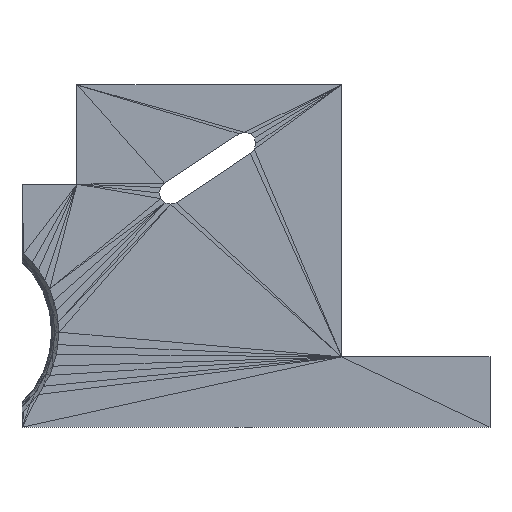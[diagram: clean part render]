
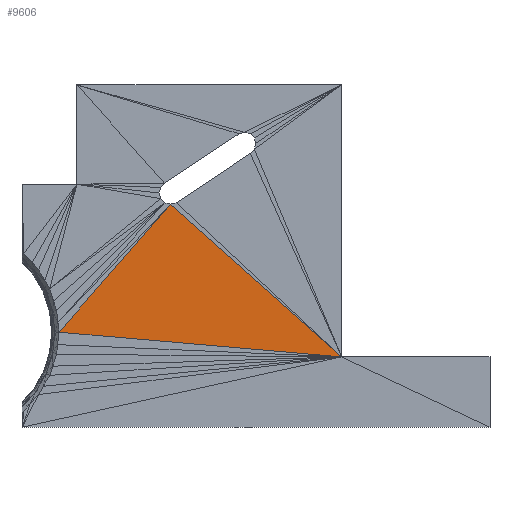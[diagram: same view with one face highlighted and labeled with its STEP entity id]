
A CAD part, top view. The second image highlights one B-rep face of the part: STEP entity #9606.
In plain terms, the highlighted planar face has unit normal (0, 0, 1).
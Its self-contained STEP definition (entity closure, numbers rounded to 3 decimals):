
#2076 = VERTEX_POINT('',#2077);
#2077 = CARTESIAN_POINT('',(12.446,-12.7,
    3.047));
#2202 = PLANE('',#2203);
#2203 = AXIS2_PLACEMENT_3D('',#2204,#2205,#2206);
#2204 = CARTESIAN_POINT('',(1.503,-2.733,
    3.047));
#2205 = DIRECTION('',(0.,0.,1.));
#2206 = DIRECTION('',(0.,1.,0.));
#2242 = EDGE_CURVE('',#2243,#2076,#2245,.T.);
#2243 = VERTEX_POINT('',#2244);
#2244 = CARTESIAN_POINT('',(-9.525,6.89,3.047
    ));
#2245 = SURFACE_CURVE('',#2246,(#2250,#2257),.PCURVE_S1.);
#2246 = LINE('',#2247,#2248);
#2247 = CARTESIAN_POINT('',(-9.525,6.89,3.047
    ));
#2248 = VECTOR('',#2249,1.);
#2249 = DIRECTION('',(0.746,-0.666,0.));
#2250 = PCURVE('',#2202,#2251);
#2251 = DEFINITIONAL_REPRESENTATION('',(#2252),#2256);
#2252 = LINE('',#2253,#2254);
#2253 = CARTESIAN_POINT('',(9.622,11.028));
#2254 = VECTOR('',#2255,1.);
#2255 = DIRECTION('',(-0.666,-0.746));
#2256 = ( GEOMETRIC_REPRESENTATION_CONTEXT(2) 
PARAMETRIC_REPRESENTATION_CONTEXT() REPRESENTATION_CONTEXT('2D SPACE',''
  ) );
#2257 = PCURVE('',#2258,#2263);
#2258 = PLANE('',#2259);
#2259 = AXIS2_PLACEMENT_3D('',#2260,#2261,#2262);
#2260 = CARTESIAN_POINT('',(-6.022,-5.922,
    3.047));
#2261 = DIRECTION('',(0.,0.,1.));
#2262 = DIRECTION('',(1.,0.,-0.));
#2263 = DEFINITIONAL_REPRESENTATION('',(#2264),#2267);
#2264 = B_SPLINE_CURVE_WITH_KNOTS('',1,(#2265,#2266),.UNSPECIFIED.,.F.,
  .F.,(2,2),(0.,29.436),.PIECEWISE_BEZIER_KNOTS.);
#2265 = CARTESIAN_POINT('',(-3.503,12.811));
#2266 = CARTESIAN_POINT('',(18.468,-6.778));
#2267 = ( GEOMETRIC_REPRESENTATION_CONTEXT(2) 
PARAMETRIC_REPRESENTATION_CONTEXT() REPRESENTATION_CONTEXT('2D SPACE',''
  ) );
#3751 = VERTEX_POINT('',#3752);
#3752 = CARTESIAN_POINT('',(-23.837,-9.525,3.047
    ));
#3766 = PLANE('',#3767);
#3767 = AXIS2_PLACEMENT_3D('',#3768,#3769,#3770);
#3768 = CARTESIAN_POINT('',(-6.131,-11.488,
    3.047));
#3769 = DIRECTION('',(0.,0.,1.));
#3770 = DIRECTION('',(0.,1.,0.));
#8823 = PLANE('',#8824);
#8824 = AXIS2_PLACEMENT_3D('',#8825,#8826,#8827);
#8825 = CARTESIAN_POINT('',(-16.915,-1.238,
    3.047));
#8826 = DIRECTION('',(0.,0.,1.));
#8827 = DIRECTION('',(1.,0.,-0.));
#9245 = EDGE_CURVE('',#3751,#2243,#9246,.T.);
#9246 = SURFACE_CURVE('',#9247,(#9251,#9258),.PCURVE_S1.);
#9247 = LINE('',#9248,#9249);
#9248 = CARTESIAN_POINT('',(-23.837,-9.525,3.047
    ));
#9249 = VECTOR('',#9250,1.);
#9250 = DIRECTION('',(0.657,0.754,0.));
#9251 = PCURVE('',#8823,#9252);
#9252 = DEFINITIONAL_REPRESENTATION('',(#9253),#9257);
#9253 = LINE('',#9254,#9255);
#9254 = CARTESIAN_POINT('',(-6.922,-8.287));
#9255 = VECTOR('',#9256,1.);
#9256 = DIRECTION('',(0.657,0.754));
#9257 = ( GEOMETRIC_REPRESENTATION_CONTEXT(2) 
PARAMETRIC_REPRESENTATION_CONTEXT() REPRESENTATION_CONTEXT('2D SPACE',''
  ) );
#9258 = PCURVE('',#2258,#9259);
#9259 = DEFINITIONAL_REPRESENTATION('',(#9260),#9263);
#9260 = B_SPLINE_CURVE_WITH_KNOTS('',1,(#9261,#9262),.UNSPECIFIED.,.F.,
  .F.,(2,2),(0.,21.778),.PIECEWISE_BEZIER_KNOTS.);
#9261 = CARTESIAN_POINT('',(-17.815,-3.603));
#9262 = CARTESIAN_POINT('',(-3.503,12.811));
#9263 = ( GEOMETRIC_REPRESENTATION_CONTEXT(2) 
PARAMETRIC_REPRESENTATION_CONTEXT() REPRESENTATION_CONTEXT('2D SPACE',''
  ) );
#9606 = ADVANCED_FACE('',(#9607),#2258,.T.);
#9607 = FACE_BOUND('',#9608,.T.);
#9608 = EDGE_LOOP('',(#9609,#9610,#9630));
#9609 = ORIENTED_EDGE('',*,*,#9245,.F.);
#9610 = ORIENTED_EDGE('',*,*,#9611,.T.);
#9611 = EDGE_CURVE('',#3751,#2076,#9612,.T.);
#9612 = SURFACE_CURVE('',#9613,(#9617,#9624),.PCURVE_S1.);
#9613 = LINE('',#9614,#9615);
#9614 = CARTESIAN_POINT('',(-23.837,-9.525,3.047
    ));
#9615 = VECTOR('',#9616,1.);
#9616 = DIRECTION('',(0.996,-0.087,0.));
#9617 = PCURVE('',#2258,#9618);
#9618 = DEFINITIONAL_REPRESENTATION('',(#9619),#9623);
#9619 = LINE('',#9620,#9621);
#9620 = CARTESIAN_POINT('',(-17.815,-3.603));
#9621 = VECTOR('',#9622,1.);
#9622 = DIRECTION('',(0.996,-0.087));
#9623 = ( GEOMETRIC_REPRESENTATION_CONTEXT(2) 
PARAMETRIC_REPRESENTATION_CONTEXT() REPRESENTATION_CONTEXT('2D SPACE',''
  ) );
#9624 = PCURVE('',#3766,#9625);
#9625 = DEFINITIONAL_REPRESENTATION('',(#9626),#9629);
#9626 = B_SPLINE_CURVE_WITH_KNOTS('',1,(#9627,#9628),.UNSPECIFIED.,.F.,
  .F.,(2,2),(0.,36.422),.PIECEWISE_BEZIER_KNOTS.);
#9627 = CARTESIAN_POINT('',(1.963,17.706));
#9628 = CARTESIAN_POINT('',(-1.212,-18.577));
#9629 = ( GEOMETRIC_REPRESENTATION_CONTEXT(2) 
PARAMETRIC_REPRESENTATION_CONTEXT() REPRESENTATION_CONTEXT('2D SPACE',''
  ) );
#9630 = ORIENTED_EDGE('',*,*,#2242,.F.);
